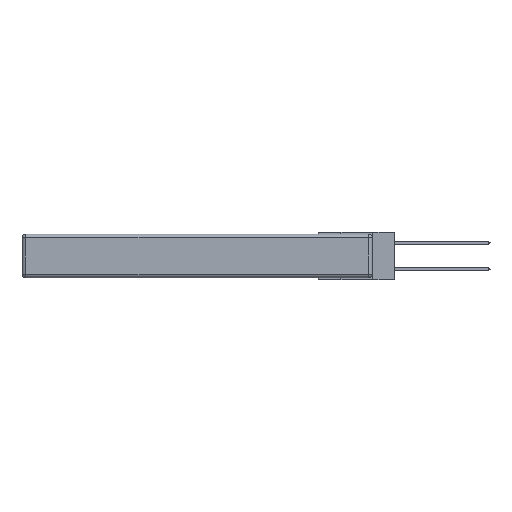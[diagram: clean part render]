
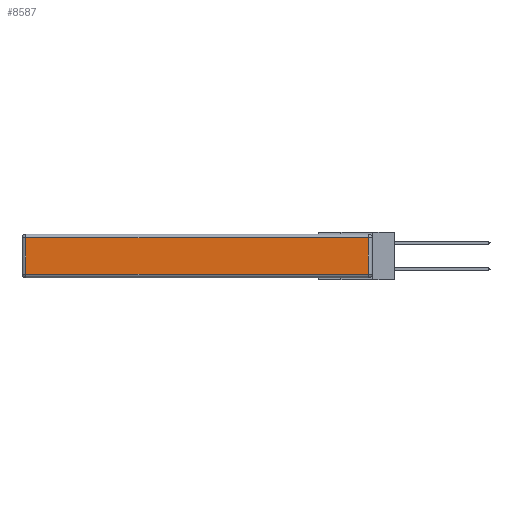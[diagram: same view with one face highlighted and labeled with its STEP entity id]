
A CAD part, left-side view. The second image highlights one B-rep face of the part: STEP entity #8587.
In plain terms, the highlighted planar face has unit normal (-1, 0, 0).
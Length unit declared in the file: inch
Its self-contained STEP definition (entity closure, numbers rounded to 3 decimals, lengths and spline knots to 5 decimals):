
#153 = EDGE_CURVE ( 'NONE', #13484, #6762, #12270, .T. ) ;
#386 = VECTOR ( 'NONE', #1261, 39.37008 ) ;
#428 = PLANE ( 'NONE',  #446 ) ;
#446 = AXIS2_PLACEMENT_3D ( 'NONE', #2505, #8040, #12222 ) ;
#601 = CARTESIAN_POINT ( 'NONE',  ( 0., 0.03, -0.343 ) ) ;
#766 = EDGE_LOOP ( 'NONE', ( #12370, #1827, #4574, #11582 ) ) ;
#875 = LINE ( 'NONE', #6625, #386 ) ;
#886 = FACE_OUTER_BOUND ( 'NONE', #766, .T. ) ;
#1261 = DIRECTION ( 'NONE',  ( 0., -1., 0. ) ) ;
#1558 = EDGE_CURVE ( 'NONE', #10875, #6453, #875, .T. ) ;
#1827 = ORIENTED_EDGE ( 'NONE', *, *, #7926, .T. ) ;
#2237 = CARTESIAN_POINT ( 'NONE',  ( 0., 2.72, -0.313 ) ) ;
#2505 = CARTESIAN_POINT ( 'NONE',  ( 0., 0., -0.343 ) ) ;
#3913 = CARTESIAN_POINT ( 'NONE',  ( 0., 2.72, -0.03 ) ) ;
#4387 = LINE ( 'NONE', #12203, #12690 ) ;
#4529 = CARTESIAN_POINT ( 'NONE',  ( 0., 0.03, -0.313 ) ) ;
#4574 = ORIENTED_EDGE ( 'NONE', *, *, #153, .T. ) ;
#4728 = DIRECTION ( 'NONE',  ( 0., 0., -1. ) ) ;
#5322 = DIRECTION ( 'NONE',  ( 0., 1., 0. ) ) ;
#6453 = VERTEX_POINT ( 'NONE', #4529 ) ;
#6625 = CARTESIAN_POINT ( 'NONE',  ( 0., 0., -0.313 ) ) ;
#6762 = VERTEX_POINT ( 'NONE', #3913 ) ;
#6927 = VECTOR ( 'NONE', #7987, 39.37008 ) ;
#7251 = CARTESIAN_POINT ( 'NONE',  ( 0., 0.03, -0.03 ) ) ;
#7926 = EDGE_CURVE ( 'NONE', #6453, #13484, #10133, .T. ) ;
#7987 = DIRECTION ( 'NONE',  ( 0., 0., 1. ) ) ;
#8040 = DIRECTION ( 'NONE',  ( -1., 0., 0. ) ) ;
#8207 = EDGE_CURVE ( 'NONE', #6762, #10875, #4387, .T. ) ;
#8240 = VECTOR ( 'NONE', #5322, 39.37008 ) ;
#8587 = ADVANCED_FACE ( 'NONE', ( #886 ), #428, .T. ) ;
#10133 = LINE ( 'NONE', #601, #6927 ) ;
#10875 = VERTEX_POINT ( 'NONE', #2237 ) ;
#11582 = ORIENTED_EDGE ( 'NONE', *, *, #8207, .T. ) ;
#11798 = CARTESIAN_POINT ( 'NONE',  ( 0., 2.75, -0.03 ) ) ;
#12203 = CARTESIAN_POINT ( 'NONE',  ( 0., 2.72, -0.343 ) ) ;
#12222 = DIRECTION ( 'NONE',  ( 0., 0., 1. ) ) ;
#12270 = LINE ( 'NONE', #11798, #8240 ) ;
#12370 = ORIENTED_EDGE ( 'NONE', *, *, #1558, .T. ) ;
#12690 = VECTOR ( 'NONE', #4728, 39.37008 ) ;
#13484 = VERTEX_POINT ( 'NONE', #7251 ) ;
